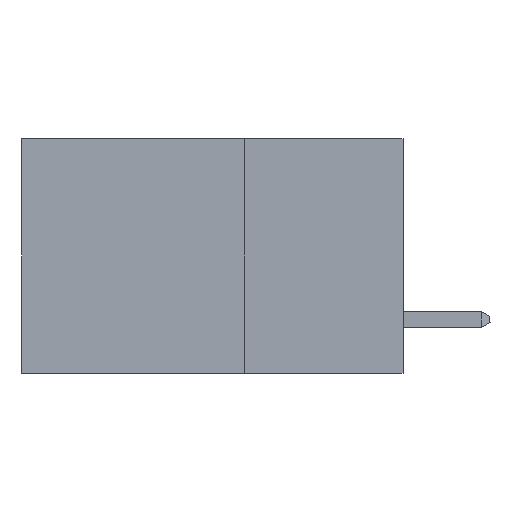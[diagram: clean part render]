
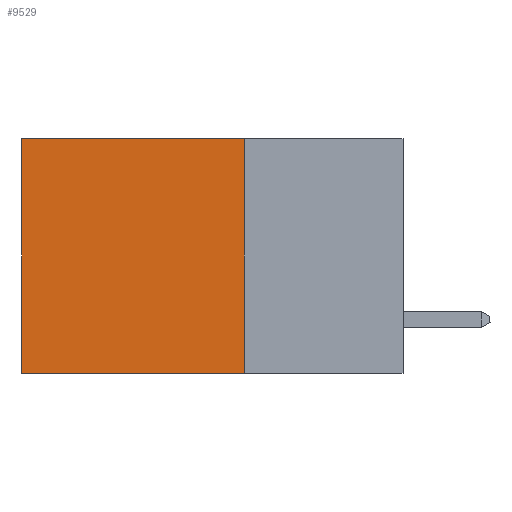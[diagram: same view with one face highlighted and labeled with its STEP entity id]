
A CAD part, left-side view. The second image highlights one B-rep face of the part: STEP entity #9529.
In plain terms, the highlighted planar face has unit normal (-1, 0, 0).
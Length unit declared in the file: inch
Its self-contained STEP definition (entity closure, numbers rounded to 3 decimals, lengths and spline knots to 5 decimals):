
#154 = DIRECTION ( 'NONE',  ( 0., 0., -1. ) ) ;
#1557 = CARTESIAN_POINT ( 'NONE',  ( 0.2875, 0.6, 0. ) ) ;
#1560 = VECTOR ( 'NONE', #154, 39.37008 ) ;
#2933 = DIRECTION ( 'NONE',  ( 0., 0., -1. ) ) ;
#4162 = ORIENTED_EDGE ( 'NONE', *, *, #11329, .T. ) ;
#4305 = VERTEX_POINT ( 'NONE', #13212 ) ;
#4634 = LINE ( 'NONE', #6454, #11593 ) ;
#4668 = DIRECTION ( 'NONE',  ( 0., 1., 0. ) ) ;
#6454 = CARTESIAN_POINT ( 'NONE',  ( 0.2875, 0.25, 0. ) ) ;
#7402 = CARTESIAN_POINT ( 'NONE',  ( 0.2875, 0.25, 0. ) ) ;
#7651 = VERTEX_POINT ( 'NONE', #7402 ) ;
#7735 = CARTESIAN_POINT ( 'NONE',  ( 0.2875, 0.6, -0.37 ) ) ;
#7819 = ORIENTED_EDGE ( 'NONE', *, *, #8205, .T. ) ;
#8205 = EDGE_CURVE ( 'NONE', #10095, #14607, #16328, .T. ) ;
#8852 = CARTESIAN_POINT ( 'NONE',  ( 0.2875, 0.25, -0.37 ) ) ;
#9529 = ADVANCED_FACE ( 'NONE', ( #9557 ), #9876, .F. ) ;
#9557 = FACE_OUTER_BOUND ( 'NONE', #12194, .T. ) ;
#9817 = DIRECTION ( 'NONE',  ( 0., 1., 0. ) ) ;
#9876 = PLANE ( 'NONE',  #13607 ) ;
#10095 = VERTEX_POINT ( 'NONE', #11050 ) ;
#10373 = VECTOR ( 'NONE', #9817, 39.37008 ) ;
#10653 = DIRECTION ( 'NONE',  ( 0., 0., -1. ) ) ;
#10984 = LINE ( 'NONE', #13929, #10373 ) ;
#11050 = CARTESIAN_POINT ( 'NONE',  ( 0.2875, 0.6, 0. ) ) ;
#11246 = DIRECTION ( 'NONE',  ( 1., 0., 0. ) ) ;
#11329 = EDGE_CURVE ( 'NONE', #7651, #10095, #10984, .T. ) ;
#11593 = VECTOR ( 'NONE', #10653, 39.37008 ) ;
#12194 = EDGE_LOOP ( 'NONE', ( #7819, #12706, #16886, #4162 ) ) ;
#12444 = VECTOR ( 'NONE', #4668, 39.37008 ) ;
#12706 = ORIENTED_EDGE ( 'NONE', *, *, #17246, .F. ) ;
#13212 = CARTESIAN_POINT ( 'NONE',  ( 0.2875, 0.25, -0.37 ) ) ;
#13308 = LINE ( 'NONE', #8852, #12444 ) ;
#13607 = AXIS2_PLACEMENT_3D ( 'NONE', #15383, #11246, #2933 ) ;
#13929 = CARTESIAN_POINT ( 'NONE',  ( 0.2875, 0.25, 0. ) ) ;
#14607 = VERTEX_POINT ( 'NONE', #7735 ) ;
#15383 = CARTESIAN_POINT ( 'NONE',  ( 0.2875, 0.25, 0. ) ) ;
#16328 = LINE ( 'NONE', #1557, #1560 ) ;
#16832 = EDGE_CURVE ( 'NONE', #7651, #4305, #4634, .T. ) ;
#16886 = ORIENTED_EDGE ( 'NONE', *, *, #16832, .F. ) ;
#17246 = EDGE_CURVE ( 'NONE', #4305, #14607, #13308, .T. ) ;
